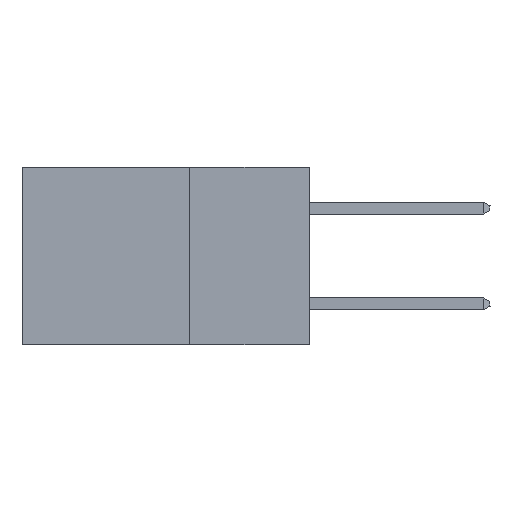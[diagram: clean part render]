
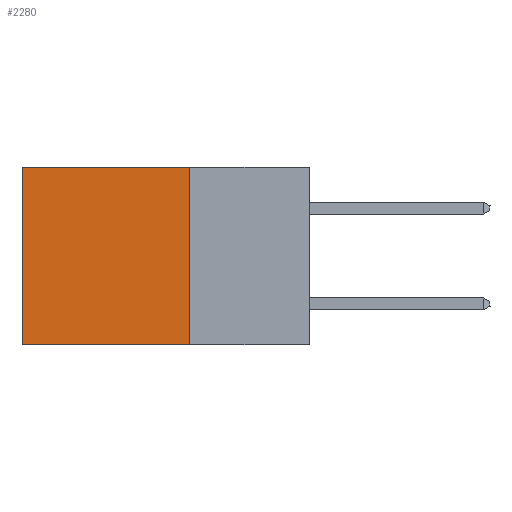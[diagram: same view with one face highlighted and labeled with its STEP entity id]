
A CAD part, left-side view. The second image highlights one B-rep face of the part: STEP entity #2280.
In plain terms, the highlighted planar face has unit normal (-1, 0, 0).
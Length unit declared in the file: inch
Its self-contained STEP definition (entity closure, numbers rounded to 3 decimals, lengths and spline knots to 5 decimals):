
#557 = CARTESIAN_POINT ( 'NONE',  ( 0.2875, 0.6, 0. ) ) ;
#591 = EDGE_LOOP ( 'NONE', ( #8506, #14110, #11860, #9037 ) ) ;
#1868 = CARTESIAN_POINT ( 'NONE',  ( 0.2875, 0.25, 0. ) ) ;
#2280 = ADVANCED_FACE ( 'NONE', ( #9172 ), #9049, .F. ) ;
#2418 = CARTESIAN_POINT ( 'NONE',  ( 0.2875, 0.6, -0.37 ) ) ;
#4237 = LINE ( 'NONE', #7279, #12566 ) ;
#4720 = DIRECTION ( 'NONE',  ( 0., 0., -1. ) ) ;
#5331 = EDGE_CURVE ( 'NONE', #7895, #6705, #19268, .T. ) ;
#6705 = VERTEX_POINT ( 'NONE', #2418 ) ;
#7279 = CARTESIAN_POINT ( 'NONE',  ( 0.2875, 0.25, -0.37 ) ) ;
#7423 = DIRECTION ( 'NONE',  ( 0., 0., -1. ) ) ;
#7895 = VERTEX_POINT ( 'NONE', #557 ) ;
#8146 = CARTESIAN_POINT ( 'NONE',  ( 0.2875, 0.25, 0. ) ) ;
#8506 = ORIENTED_EDGE ( 'NONE', *, *, #5331, .T. ) ;
#9037 = ORIENTED_EDGE ( 'NONE', *, *, #16806, .T. ) ;
#9049 = PLANE ( 'NONE',  #10956 ) ;
#9128 = VERTEX_POINT ( 'NONE', #17085 ) ;
#9172 = FACE_OUTER_BOUND ( 'NONE', #591, .T. ) ;
#10726 = VECTOR ( 'NONE', #14636, 39.37008 ) ;
#10880 = LINE ( 'NONE', #19408, #14686 ) ;
#10956 = AXIS2_PLACEMENT_3D ( 'NONE', #15551, #17181, #7423 ) ;
#11860 = ORIENTED_EDGE ( 'NONE', *, *, #11909, .F. ) ;
#11909 = EDGE_CURVE ( 'NONE', #18546, #9128, #10880, .T. ) ;
#12566 = VECTOR ( 'NONE', #18633, 39.37008 ) ;
#14110 = ORIENTED_EDGE ( 'NONE', *, *, #16453, .F. ) ;
#14636 = DIRECTION ( 'NONE',  ( 0., 1., 0. ) ) ;
#14686 = VECTOR ( 'NONE', #4720, 39.37008 ) ;
#15000 = VECTOR ( 'NONE', #15654, 39.37008 ) ;
#15023 = LINE ( 'NONE', #8146, #10726 ) ;
#15551 = CARTESIAN_POINT ( 'NONE',  ( 0.2875, 0.25, 0. ) ) ;
#15654 = DIRECTION ( 'NONE',  ( 0., 0., -1. ) ) ;
#16453 = EDGE_CURVE ( 'NONE', #9128, #6705, #4237, .T. ) ;
#16806 = EDGE_CURVE ( 'NONE', #18546, #7895, #15023, .T. ) ;
#17085 = CARTESIAN_POINT ( 'NONE',  ( 0.2875, 0.25, -0.37 ) ) ;
#17181 = DIRECTION ( 'NONE',  ( 1., 0., 0. ) ) ;
#17207 = CARTESIAN_POINT ( 'NONE',  ( 0.2875, 0.6, 0. ) ) ;
#18546 = VERTEX_POINT ( 'NONE', #1868 ) ;
#18633 = DIRECTION ( 'NONE',  ( 0., 1., 0. ) ) ;
#19268 = LINE ( 'NONE', #17207, #15000 ) ;
#19408 = CARTESIAN_POINT ( 'NONE',  ( 0.2875, 0.25, 0. ) ) ;
